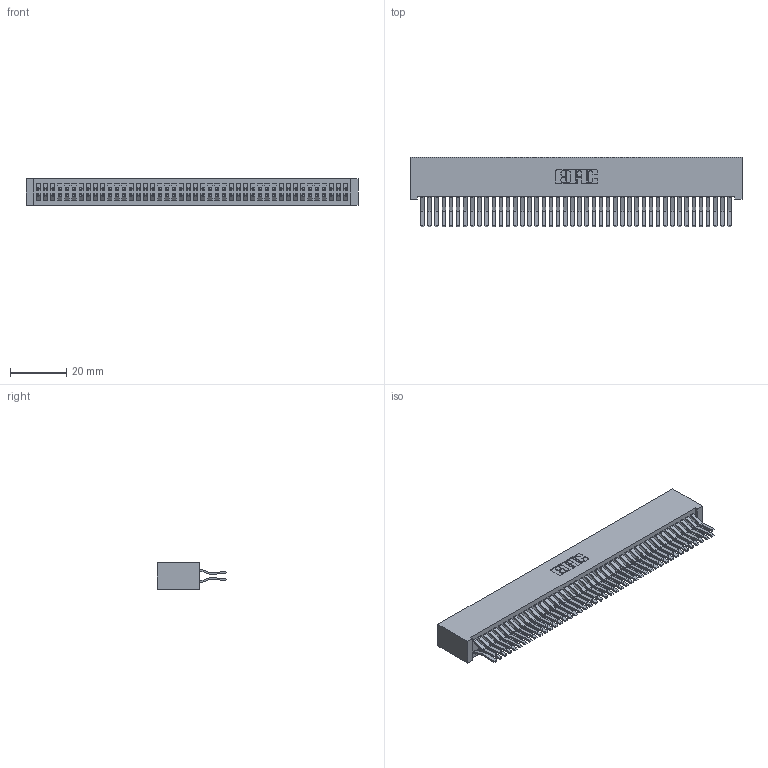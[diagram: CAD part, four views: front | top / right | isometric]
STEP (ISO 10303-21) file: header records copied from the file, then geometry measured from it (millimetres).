
FILE_DESCRIPTION (( 'STEP AP203' ), '1' );
FILE_NAME ('342-088-560-201.STEP', '2018-08-14T00:46:07', ( '' ), ( '' ), 'SwSTEP 2.0', 'SolidWorks 2016', '' );
FILE_SCHEMA (( 'CONFIG_CONTROL_DESIGN' ));
Length unit declared in the file: inch
Products named in the file (3): 342 Part_Lugless; 345-292-001_560 Tail; 342-088-560-201
Assembly tree (89 placements, depth 2):
  342-088-560-201
    342 Part_Lugless
    345-292-001_560 Tail  x88
Bounding box: 118.01 x 24.78 x 9.4 mm (x, y, z)
Volume: 11629.8 mm3; surface area: 20811.2 mm2
Topology: 89 solids, 89 shells, 4854 faces, 14443 edges, 9510 vertices
Faces by surface type: plane 3230, cylinder 1624
Entity records: 27727 total; most frequent: CARTESIAN_POINT 4590, ORIENTED_EDGE 4526, DIRECTION 3915, EDGE_CURVE 2263, VECTOR 2139, LINE 2139, VERTEX_POINT 1506, AXIS2_PLACEMENT_3D 888
